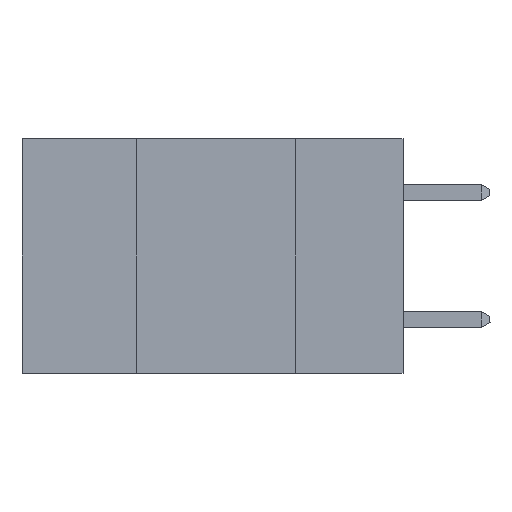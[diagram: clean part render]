
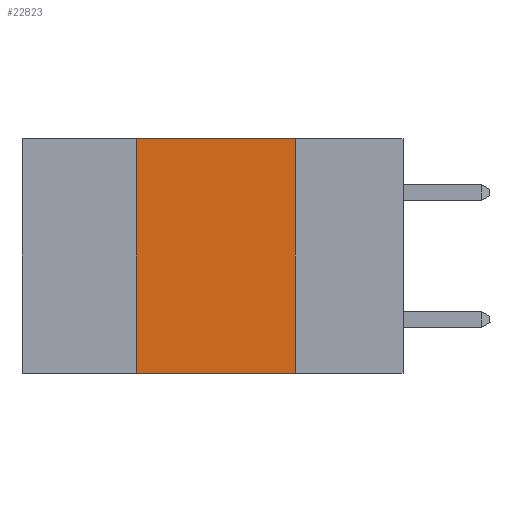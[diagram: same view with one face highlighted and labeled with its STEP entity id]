
A CAD part, left-side view. The second image highlights one B-rep face of the part: STEP entity #22823.
In plain terms, the highlighted planar face has unit normal (-1, 0, 0).
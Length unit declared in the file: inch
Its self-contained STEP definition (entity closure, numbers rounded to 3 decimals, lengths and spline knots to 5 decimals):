
#2271 = EDGE_CURVE ( 'NONE', #24765, #14267, #26223, .T. ) ;
#3119 = EDGE_CURVE ( 'NONE', #24765, #11218, #10326, .T. ) ;
#4540 = ORIENTED_EDGE ( 'NONE', *, *, #32588, .F. ) ;
#6461 = VECTOR ( 'NONE', #28237, 39.37008 ) ;
#6874 = ORIENTED_EDGE ( 'NONE', *, *, #3119, .T. ) ;
#7648 = VECTOR ( 'NONE', #36605, 39.37008 ) ;
#9965 = CARTESIAN_POINT ( 'NONE',  ( 0., 0.6, -0.37 ) ) ;
#10326 = LINE ( 'NONE', #9965, #30522 ) ;
#10867 = ORIENTED_EDGE ( 'NONE', *, *, #22614, .F. ) ;
#10977 = CARTESIAN_POINT ( 'NONE',  ( 0., 0.17, 0. ) ) ;
#11218 = VERTEX_POINT ( 'NONE', #17339 ) ;
#14267 = VERTEX_POINT ( 'NONE', #31904 ) ;
#15041 = DIRECTION ( 'NONE',  ( 0., 0., -1. ) ) ;
#15183 = VERTEX_POINT ( 'NONE', #24204 ) ;
#17339 = CARTESIAN_POINT ( 'NONE',  ( 0., 0.17, -0.37 ) ) ;
#18094 = VECTOR ( 'NONE', #26551, 39.37008 ) ;
#18381 = PLANE ( 'NONE',  #33791 ) ;
#18588 = CARTESIAN_POINT ( 'NONE',  ( 0., 0.42, 0. ) ) ;
#22614 = EDGE_CURVE ( 'NONE', #14267, #15183, #31429, .T. ) ;
#22823 = ADVANCED_FACE ( 'NONE', ( #31390 ), #18381, .F. ) ;
#23025 = EDGE_LOOP ( 'NONE', ( #4540, #10867, #38709, #6874 ) ) ;
#24204 = CARTESIAN_POINT ( 'NONE',  ( 0., 0.17, 0. ) ) ;
#24765 = VERTEX_POINT ( 'NONE', #39727 ) ;
#24873 = CARTESIAN_POINT ( 'NONE',  ( 0., 0.6, 0. ) ) ;
#25005 = DIRECTION ( 'NONE',  ( 1., 0., 0. ) ) ;
#26223 = LINE ( 'NONE', #18588, #6461 ) ;
#26551 = DIRECTION ( 'NONE',  ( 0., -1., 0. ) ) ;
#26896 = LINE ( 'NONE', #10977, #7648 ) ;
#28237 = DIRECTION ( 'NONE',  ( 0., 0., 1. ) ) ;
#30522 = VECTOR ( 'NONE', #32298, 39.37008 ) ;
#31390 = FACE_OUTER_BOUND ( 'NONE', #23025, .T. ) ;
#31429 = LINE ( 'NONE', #39103, #18094 ) ;
#31904 = CARTESIAN_POINT ( 'NONE',  ( 0., 0.42, 0. ) ) ;
#32298 = DIRECTION ( 'NONE',  ( 0., -1., 0. ) ) ;
#32588 = EDGE_CURVE ( 'NONE', #15183, #11218, #26896, .T. ) ;
#33791 = AXIS2_PLACEMENT_3D ( 'NONE', #24873, #25005, #15041 ) ;
#36605 = DIRECTION ( 'NONE',  ( 0., 0., -1. ) ) ;
#38709 = ORIENTED_EDGE ( 'NONE', *, *, #2271, .F. ) ;
#39103 = CARTESIAN_POINT ( 'NONE',  ( 0., 0.6, 0. ) ) ;
#39727 = CARTESIAN_POINT ( 'NONE',  ( 0., 0.42, -0.37 ) ) ;
